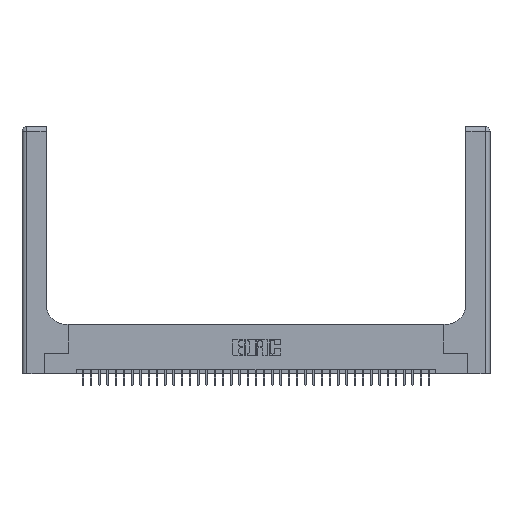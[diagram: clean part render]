
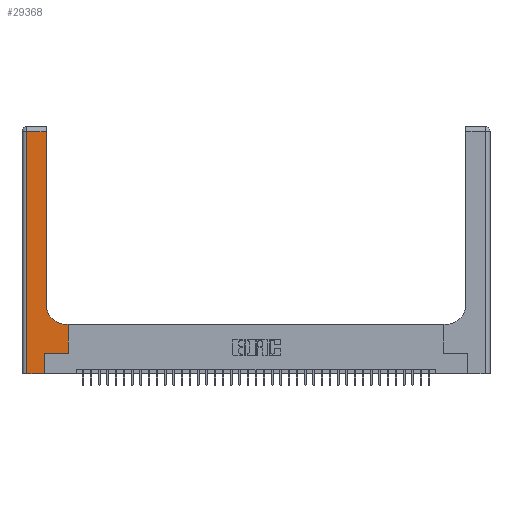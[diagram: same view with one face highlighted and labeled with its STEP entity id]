
A CAD part, top view. The second image highlights one B-rep face of the part: STEP entity #29368.
In plain terms, the highlighted planar face has unit normal (0, 0, 1).
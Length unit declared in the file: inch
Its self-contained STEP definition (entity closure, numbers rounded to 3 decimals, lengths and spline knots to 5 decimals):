
#34 = VECTOR ( 'NONE', #5898, 39.37008 ) ;
#1140 = DIRECTION ( 'NONE',  ( 0., 1., 0. ) ) ;
#1522 = CARTESIAN_POINT ( 'NONE',  ( 0.269, 0.25, 0.37 ) ) ;
#1780 = EDGE_LOOP ( 'NONE', ( #4694, #27127, #13827, #12434, #11121, #28698, #14154, #3039, #9820 ) ) ;
#2112 = VECTOR ( 'NONE', #8413, 39.37008 ) ;
#2451 = EDGE_CURVE ( 'NONE', #16776, #4444, #32885, .T. ) ;
#3039 = ORIENTED_EDGE ( 'NONE', *, *, #5813, .T. ) ;
#3413 = DIRECTION ( 'NONE',  ( 1., 0., 0. ) ) ;
#3699 = LINE ( 'NONE', #27723, #26674 ) ;
#3931 = DIRECTION ( 'NONE',  ( 1., 0., 0. ) ) ;
#4093 = VERTEX_POINT ( 'NONE', #11643 ) ;
#4258 = LINE ( 'NONE', #22938, #28546 ) ;
#4444 = VERTEX_POINT ( 'NONE', #14747 ) ;
#4694 = ORIENTED_EDGE ( 'NONE', *, *, #27633, .T. ) ;
#5813 = EDGE_CURVE ( 'NONE', #19094, #4093, #15539, .T. ) ;
#5898 = DIRECTION ( 'NONE',  ( 0., -1., 0. ) ) ;
#5907 = VECTOR ( 'NONE', #3413, 39.37008 ) ;
#6123 = EDGE_CURVE ( 'NONE', #4444, #27651, #17666, .T. ) ;
#7064 = VERTEX_POINT ( 'NONE', #27010 ) ;
#7478 = VERTEX_POINT ( 'NONE', #24755 ) ;
#7791 = DIRECTION ( 'NONE',  ( 0., 0., -1. ) ) ;
#8413 = DIRECTION ( 'NONE',  ( 1., 0., 0. ) ) ;
#9820 = ORIENTED_EDGE ( 'NONE', *, *, #37030, .T. ) ;
#10597 = VERTEX_POINT ( 'NONE', #1522 ) ;
#11121 = ORIENTED_EDGE ( 'NONE', *, *, #26376, .T. ) ;
#11643 = CARTESIAN_POINT ( 'NONE',  ( 0.5415, 0.6, 0.37 ) ) ;
#11995 = EDGE_CURVE ( 'NONE', #10597, #18657, #30383, .T. ) ;
#12434 = ORIENTED_EDGE ( 'NONE', *, *, #6123, .T. ) ;
#13510 = CARTESIAN_POINT ( 'NONE',  ( 0., 3., 0.37 ) ) ;
#13827 = ORIENTED_EDGE ( 'NONE', *, *, #2451, .T. ) ;
#14154 = ORIENTED_EDGE ( 'NONE', *, *, #25766, .T. ) ;
#14666 = VECTOR ( 'NONE', #27547, 39.37008 ) ;
#14747 = CARTESIAN_POINT ( 'NONE',  ( 0.06, 0., 0.37 ) ) ;
#14973 = VECTOR ( 'NONE', #26778, 39.37008 ) ;
#15166 = LINE ( 'NONE', #15560, #14973 ) ;
#15539 = LINE ( 'NONE', #36827, #14666 ) ;
#15560 = CARTESIAN_POINT ( 'NONE',  ( 0.5585, 0.25, 0.37 ) ) ;
#15610 = CARTESIAN_POINT ( 'NONE',  ( 0.269, 0.25, 0.37 ) ) ;
#16086 = PLANE ( 'NONE',  #16763 ) ;
#16763 = AXIS2_PLACEMENT_3D ( 'NONE', #13510, #7791, #21977 ) ;
#16776 = VERTEX_POINT ( 'NONE', #20648 ) ;
#17666 = LINE ( 'NONE', #38353, #2112 ) ;
#18292 = CARTESIAN_POINT ( 'NONE',  ( 0.06, 3., 0.37 ) ) ;
#18487 = CARTESIAN_POINT ( 'NONE',  ( 0.5415, 0.85, 0.37 ) ) ;
#18627 = CARTESIAN_POINT ( 'NONE',  ( 0.5585, 0.25, 0.37 ) ) ;
#18657 = VERTEX_POINT ( 'NONE', #18627 ) ;
#18990 = EDGE_CURVE ( 'NONE', #7064, #16776, #4258, .T. ) ;
#19094 = VERTEX_POINT ( 'NONE', #23329 ) ;
#20372 = DIRECTION ( 'NONE',  ( -1., 0., 0. ) ) ;
#20648 = CARTESIAN_POINT ( 'NONE',  ( 0.06, 2.94, 0.37 ) ) ;
#21164 = CARTESIAN_POINT ( 'NONE',  ( 0.269, 0., 0.37 ) ) ;
#21444 = DIRECTION ( 'NONE',  ( 0., 0., -1. ) ) ;
#21977 = DIRECTION ( 'NONE',  ( -1., 0., 0. ) ) ;
#22004 = CARTESIAN_POINT ( 'NONE',  ( 0.2915, 3., 0.37 ) ) ;
#22176 = FACE_OUTER_BOUND ( 'NONE', #1780, .T. ) ;
#22938 = CARTESIAN_POINT ( 'NONE',  ( 0., 2.94, 0.37 ) ) ;
#23329 = CARTESIAN_POINT ( 'NONE',  ( 0.5585, 0.6, 0.37 ) ) ;
#24755 = CARTESIAN_POINT ( 'NONE',  ( 0.2915, 0.85, 0.37 ) ) ;
#25766 = EDGE_CURVE ( 'NONE', #18657, #19094, #15166, .T. ) ;
#26376 = EDGE_CURVE ( 'NONE', #27651, #10597, #3699, .T. ) ;
#26674 = VECTOR ( 'NONE', #1140, 39.37008 ) ;
#26778 = DIRECTION ( 'NONE',  ( 0., 1., 0. ) ) ;
#27003 = AXIS2_PLACEMENT_3D ( 'NONE', #18487, #21444, #3931 ) ;
#27010 = CARTESIAN_POINT ( 'NONE',  ( 0.2915, 2.94, 0.37 ) ) ;
#27127 = ORIENTED_EDGE ( 'NONE', *, *, #18990, .T. ) ;
#27547 = DIRECTION ( 'NONE',  ( -1., 0., 0. ) ) ;
#27633 = EDGE_CURVE ( 'NONE', #7478, #7064, #36995, .T. ) ;
#27651 = VERTEX_POINT ( 'NONE', #21164 ) ;
#27723 = CARTESIAN_POINT ( 'NONE',  ( 0.269, 0., 0.37 ) ) ;
#28546 = VECTOR ( 'NONE', #20372, 39.37008 ) ;
#28698 = ORIENTED_EDGE ( 'NONE', *, *, #11995, .T. ) ;
#29368 = ADVANCED_FACE ( 'NONE', ( #22176 ), #16086, .F. ) ;
#30383 = LINE ( 'NONE', #15610, #5907 ) ;
#32885 = LINE ( 'NONE', #18292, #34 ) ;
#34034 = DIRECTION ( 'NONE',  ( 0., 1., 0. ) ) ;
#34593 = CIRCLE ( 'NONE', #27003, 0.25 ) ;
#36827 = CARTESIAN_POINT ( 'NONE',  ( 0.2915, 0.6, 0.37 ) ) ;
#36995 = LINE ( 'NONE', #22004, #38691 ) ;
#37030 = EDGE_CURVE ( 'NONE', #4093, #7478, #34593, .T. ) ;
#38353 = CARTESIAN_POINT ( 'NONE',  ( 0., 0., 0.37 ) ) ;
#38691 = VECTOR ( 'NONE', #34034, 39.37008 ) ;
